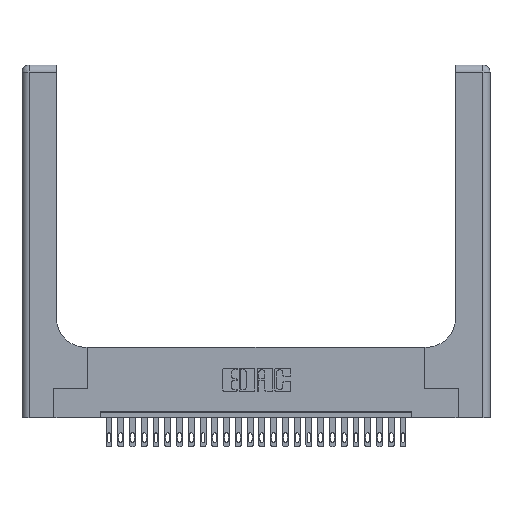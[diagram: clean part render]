
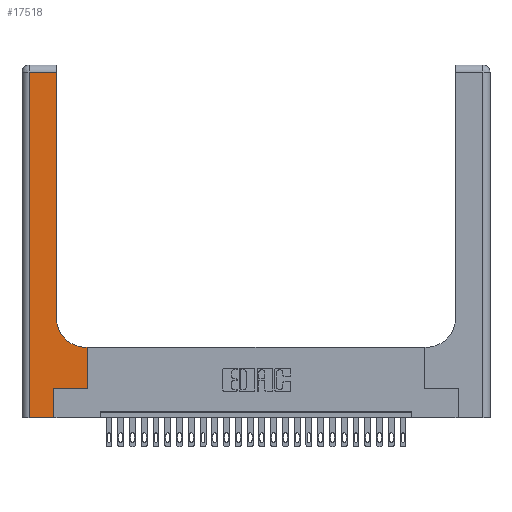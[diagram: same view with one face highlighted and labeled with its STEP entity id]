
A CAD part, top view. The second image highlights one B-rep face of the part: STEP entity #17518.
In plain terms, the highlighted planar face has unit normal (0, 0, 1).
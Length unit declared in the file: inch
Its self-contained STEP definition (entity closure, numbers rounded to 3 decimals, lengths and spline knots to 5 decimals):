
#1768 = CARTESIAN_POINT ( 'NONE',  ( 0., 3., 0.37 ) ) ;
#2187 = VERTEX_POINT ( 'NONE', #24241 ) ;
#2208 = LINE ( 'NONE', #12454, #7998 ) ;
#2551 = VERTEX_POINT ( 'NONE', #13053 ) ;
#2564 = VERTEX_POINT ( 'NONE', #2936 ) ;
#2922 = ORIENTED_EDGE ( 'NONE', *, *, #19618, .T. ) ;
#2936 = CARTESIAN_POINT ( 'NONE',  ( 0.5585, 0.6, 0.37 ) ) ;
#3127 = ORIENTED_EDGE ( 'NONE', *, *, #9679, .T. ) ;
#4049 = DIRECTION ( 'NONE',  ( 0., 1., 0. ) ) ;
#4474 = VECTOR ( 'NONE', #12091, 39.37008 ) ;
#4650 = CARTESIAN_POINT ( 'NONE',  ( 0.269, 0.25, 0.37 ) ) ;
#4753 = VERTEX_POINT ( 'NONE', #20565 ) ;
#5278 = AXIS2_PLACEMENT_3D ( 'NONE', #1768, #16201, #20372 ) ;
#5827 = CARTESIAN_POINT ( 'NONE',  ( 0.5585, 0.25, 0.37 ) ) ;
#6556 = CIRCLE ( 'NONE', #11555, 0.25 ) ;
#7341 = VERTEX_POINT ( 'NONE', #14206 ) ;
#7344 = EDGE_CURVE ( 'NONE', #7341, #2564, #18646, .T. ) ;
#7790 = DIRECTION ( 'NONE',  ( -1., 0., 0. ) ) ;
#7899 = DIRECTION ( 'NONE',  ( 0., 1., 0. ) ) ;
#7998 = VECTOR ( 'NONE', #4049, 39.37008 ) ;
#8532 = LINE ( 'NONE', #18262, #14974 ) ;
#8961 = EDGE_LOOP ( 'NONE', ( #2922, #26723, #11738, #3127, #9081, #11764, #9382, #17957, #18975 ) ) ;
#9081 = ORIENTED_EDGE ( 'NONE', *, *, #16244, .T. ) ;
#9119 = CARTESIAN_POINT ( 'NONE',  ( 0.269, 0.25, 0.37 ) ) ;
#9382 = ORIENTED_EDGE ( 'NONE', *, *, #7344, .T. ) ;
#9388 = CARTESIAN_POINT ( 'NONE',  ( 0.06, 0., 0.37 ) ) ;
#9679 = EDGE_CURVE ( 'NONE', #11443, #2551, #16914, .T. ) ;
#10014 = CARTESIAN_POINT ( 'NONE',  ( 0., 2.94, 0.37 ) ) ;
#11237 = DIRECTION ( 'NONE',  ( 1., 0., 0. ) ) ;
#11245 = LINE ( 'NONE', #10014, #4474 ) ;
#11443 = VERTEX_POINT ( 'NONE', #9388 ) ;
#11555 = AXIS2_PLACEMENT_3D ( 'NONE', #16260, #14098, #22280 ) ;
#11738 = ORIENTED_EDGE ( 'NONE', *, *, #20596, .T. ) ;
#11764 = ORIENTED_EDGE ( 'NONE', *, *, #14796, .T. ) ;
#12091 = DIRECTION ( 'NONE',  ( -1., 0., 0. ) ) ;
#12454 = CARTESIAN_POINT ( 'NONE',  ( 0.2915, 3., 0.37 ) ) ;
#12832 = VECTOR ( 'NONE', #13483, 39.37008 ) ;
#13053 = CARTESIAN_POINT ( 'NONE',  ( 0.269, 0., 0.37 ) ) ;
#13483 = DIRECTION ( 'NONE',  ( 0., -1., 0. ) ) ;
#14098 = DIRECTION ( 'NONE',  ( 0., 0., -1. ) ) ;
#14128 = PLANE ( 'NONE',  #5278 ) ;
#14206 = CARTESIAN_POINT ( 'NONE',  ( 0.5585, 0.25, 0.37 ) ) ;
#14247 = FACE_OUTER_BOUND ( 'NONE', #8961, .T. ) ;
#14712 = VERTEX_POINT ( 'NONE', #22921 ) ;
#14796 = EDGE_CURVE ( 'NONE', #22964, #7341, #15988, .T. ) ;
#14974 = VECTOR ( 'NONE', #15909, 39.37008 ) ;
#15010 = CARTESIAN_POINT ( 'NONE',  ( 0.2915, 0.85, 0.37 ) ) ;
#15513 = LINE ( 'NONE', #24565, #23350 ) ;
#15909 = DIRECTION ( 'NONE',  ( 0., 1., 0. ) ) ;
#15988 = LINE ( 'NONE', #4650, #26420 ) ;
#16201 = DIRECTION ( 'NONE',  ( 0., 0., -1. ) ) ;
#16244 = EDGE_CURVE ( 'NONE', #2551, #22964, #8532, .T. ) ;
#16260 = CARTESIAN_POINT ( 'NONE',  ( 0.5415, 0.85, 0.37 ) ) ;
#16914 = LINE ( 'NONE', #23936, #21486 ) ;
#17377 = CARTESIAN_POINT ( 'NONE',  ( 0.06, 3., 0.37 ) ) ;
#17518 = ADVANCED_FACE ( 'NONE', ( #14247 ), #14128, .F. ) ;
#17957 = ORIENTED_EDGE ( 'NONE', *, *, #23658, .T. ) ;
#18262 = CARTESIAN_POINT ( 'NONE',  ( 0.269, 0., 0.37 ) ) ;
#18646 = LINE ( 'NONE', #5827, #19940 ) ;
#18653 = VERTEX_POINT ( 'NONE', #15010 ) ;
#18975 = ORIENTED_EDGE ( 'NONE', *, *, #21910, .T. ) ;
#19548 = EDGE_CURVE ( 'NONE', #2187, #14712, #11245, .T. ) ;
#19618 = EDGE_CURVE ( 'NONE', #18653, #2187, #2208, .T. ) ;
#19940 = VECTOR ( 'NONE', #7899, 39.37008 ) ;
#20372 = DIRECTION ( 'NONE',  ( -1., 0., 0. ) ) ;
#20565 = CARTESIAN_POINT ( 'NONE',  ( 0.5415, 0.6, 0.37 ) ) ;
#20596 = EDGE_CURVE ( 'NONE', #14712, #11443, #24804, .T. ) ;
#21486 = VECTOR ( 'NONE', #11237, 39.37008 ) ;
#21910 = EDGE_CURVE ( 'NONE', #4753, #18653, #6556, .T. ) ;
#22280 = DIRECTION ( 'NONE',  ( 1., 0., 0. ) ) ;
#22921 = CARTESIAN_POINT ( 'NONE',  ( 0.06, 2.94, 0.37 ) ) ;
#22964 = VERTEX_POINT ( 'NONE', #9119 ) ;
#23350 = VECTOR ( 'NONE', #7790, 39.37008 ) ;
#23658 = EDGE_CURVE ( 'NONE', #2564, #4753, #15513, .T. ) ;
#23936 = CARTESIAN_POINT ( 'NONE',  ( 0., 0., 0.37 ) ) ;
#24241 = CARTESIAN_POINT ( 'NONE',  ( 0.2915, 2.94, 0.37 ) ) ;
#24565 = CARTESIAN_POINT ( 'NONE',  ( 0.2915, 0.6, 0.37 ) ) ;
#24804 = LINE ( 'NONE', #17377, #12832 ) ;
#25652 = DIRECTION ( 'NONE',  ( 1., 0., 0. ) ) ;
#26420 = VECTOR ( 'NONE', #25652, 39.37008 ) ;
#26723 = ORIENTED_EDGE ( 'NONE', *, *, #19548, .T. ) ;
